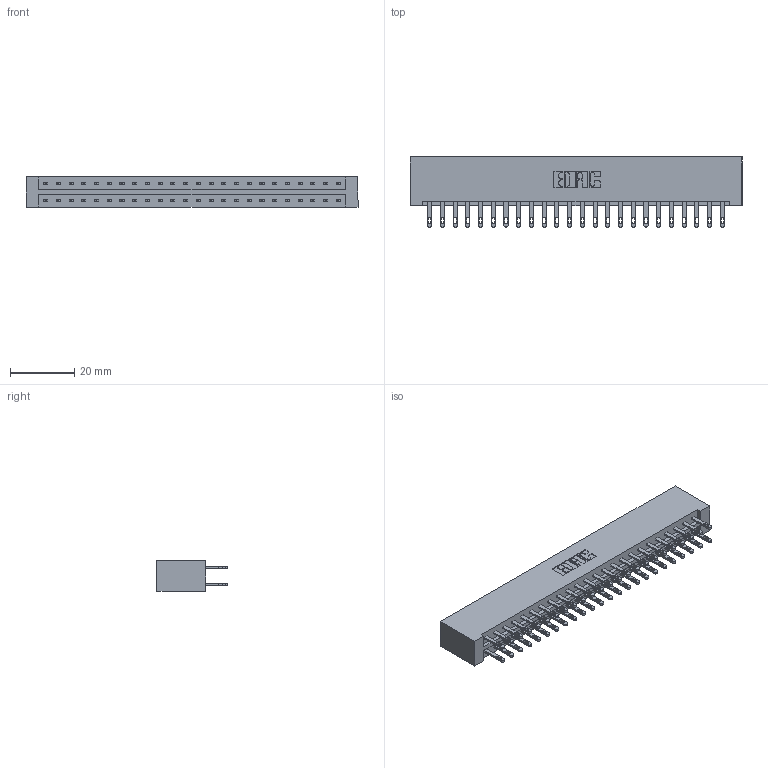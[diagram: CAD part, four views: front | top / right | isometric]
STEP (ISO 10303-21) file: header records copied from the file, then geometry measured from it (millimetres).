
FILE_DESCRIPTION (( 'STEP AP203' ), '1' );
FILE_NAME ('333-048-500-201.STEP', '2018-08-03T23:04:44', ( '' ), ( '' ), 'SwSTEP 2.0', 'SolidWorks 2016', '' );
FILE_SCHEMA (( 'CONFIG_CONTROL_DESIGN' ));
Length unit declared in the file: inch
Products named in the file (3): 333 Part_Lugless; 345-292-001_345-293-100; 333-048-500-201
Assembly tree (49 placements, depth 2):
  333-048-500-201
    333 Part_Lugless
    345-292-001_345-293-100  x48
Bounding box: 103.35 x 21.85 x 9.4 mm (x, y, z)
Volume: 11162.3 mm3; surface area: 13555.7 mm2
Topology: 49 solids, 49 shells, 2410 faces, 7343 edges, 4894 vertices
Faces by surface type: plane 1506, cylinder 904
Entity records: 17421 total; most frequent: CARTESIAN_POINT 2906, ORIENTED_EDGE 2842, DIRECTION 2509, EDGE_CURVE 1421, VECTOR 1297, LINE 1297, VERTEX_POINT 946, AXIS2_PLACEMENT_3D 606
